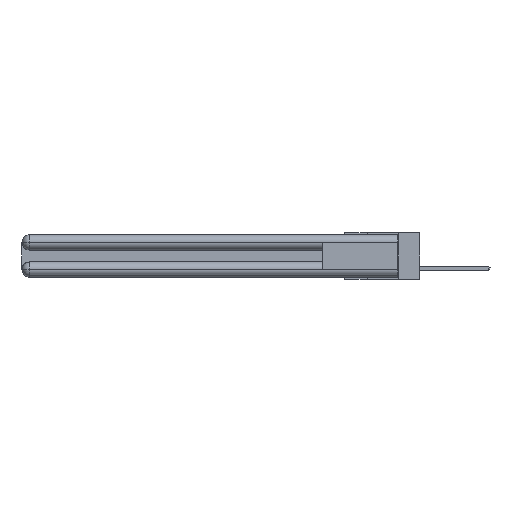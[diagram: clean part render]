
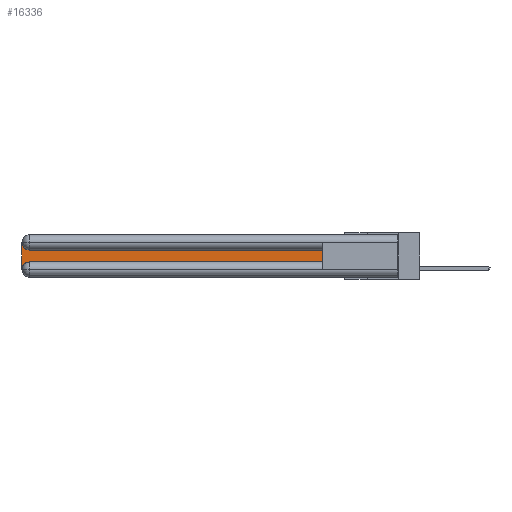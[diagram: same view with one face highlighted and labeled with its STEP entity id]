
A CAD part, left-side view. The second image highlights one B-rep face of the part: STEP entity #16336.
In plain terms, the highlighted planar face has unit normal (-1, 0, 0).
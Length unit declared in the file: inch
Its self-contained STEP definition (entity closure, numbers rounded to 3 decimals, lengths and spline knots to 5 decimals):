
#939 = VERTEX_POINT ( 'NONE', #7410 ) ;
#1721 = EDGE_CURVE ( 'NONE', #10157, #14634, #21906, .T. ) ;
#2072 = AXIS2_PLACEMENT_3D ( 'NONE', #21760, #19560, #8118 ) ;
#2104 = VERTEX_POINT ( 'NONE', #8947 ) ;
#2457 = VECTOR ( 'NONE', #24616, 39.37008 ) ;
#3689 = EDGE_LOOP ( 'NONE', ( #20193, #21967, #5775, #28191, #15033, #26736 ) ) ;
#3956 = EDGE_CURVE ( 'NONE', #939, #10157, #23600, .T. ) ;
#5775 = ORIENTED_EDGE ( 'NONE', *, *, #11467, .T. ) ;
#7410 = CARTESIAN_POINT ( 'NONE',  ( 0.075, 2.94, -0.2175 ) ) ;
#8118 = DIRECTION ( 'NONE',  ( 0., 0., -1. ) ) ;
#8134 = CARTESIAN_POINT ( 'NONE',  ( 0.075, 0.6, -0.1225 ) ) ;
#8425 = VERTEX_POINT ( 'NONE', #16467 ) ;
#8947 = CARTESIAN_POINT ( 'NONE',  ( 0.075, 3., -0.0625 ) ) ;
#10157 = VERTEX_POINT ( 'NONE', #27084 ) ;
#11119 = VECTOR ( 'NONE', #19125, 39.37008 ) ;
#11467 = EDGE_CURVE ( 'NONE', #2104, #8425, #17128, .T. ) ;
#12476 = AXIS2_PLACEMENT_3D ( 'NONE', #21191, #23612, #19287 ) ;
#13942 = VERTEX_POINT ( 'NONE', #28462 ) ;
#14634 = VERTEX_POINT ( 'NONE', #8134 ) ;
#15033 = ORIENTED_EDGE ( 'NONE', *, *, #3956, .T. ) ;
#15113 = CARTESIAN_POINT ( 'NONE',  ( 0.075, 3., -0.1225 ) ) ;
#15342 = EDGE_CURVE ( 'NONE', #8425, #939, #21113, .T. ) ;
#15667 = VECTOR ( 'NONE', #25379, 39.37008 ) ;
#16336 = ADVANCED_FACE ( 'NONE', ( #28320 ), #28887, .F. ) ;
#16467 = CARTESIAN_POINT ( 'NONE',  ( 0.075, 3., -0.2775 ) ) ;
#17128 = LINE ( 'NONE', #23083, #15667 ) ;
#17591 = CARTESIAN_POINT ( 'NONE',  ( 0.075, 0.6, -0.2175 ) ) ;
#19125 = DIRECTION ( 'NONE',  ( 0., 0., 1. ) ) ;
#19287 = DIRECTION ( 'NONE',  ( 0., 0., -1. ) ) ;
#19548 = VECTOR ( 'NONE', #29586, 39.37008 ) ;
#19560 = DIRECTION ( 'NONE',  ( 1., 0., 0. ) ) ;
#20193 = ORIENTED_EDGE ( 'NONE', *, *, #24172, .T. ) ;
#20629 = EDGE_CURVE ( 'NONE', #13942, #2104, #27631, .T. ) ;
#20967 = LINE ( 'NONE', #25072, #19548 ) ;
#21113 = CIRCLE ( 'NONE', #2072, 0.06 ) ;
#21191 = CARTESIAN_POINT ( 'NONE',  ( 0.075, 2.94, -0.0625 ) ) ;
#21760 = CARTESIAN_POINT ( 'NONE',  ( 0.075, 2.94, -0.2775 ) ) ;
#21906 = LINE ( 'NONE', #27532, #11119 ) ;
#21967 = ORIENTED_EDGE ( 'NONE', *, *, #20629, .T. ) ;
#22059 = DIRECTION ( 'NONE',  ( 1., 0., 0. ) ) ;
#23083 = CARTESIAN_POINT ( 'NONE',  ( 0.075, 3., -0.2175 ) ) ;
#23600 = LINE ( 'NONE', #17591, #2457 ) ;
#23612 = DIRECTION ( 'NONE',  ( 1., 0., 0. ) ) ;
#24172 = EDGE_CURVE ( 'NONE', #14634, #13942, #20967, .T. ) ;
#24381 = DIRECTION ( 'NONE',  ( 0., 0., -1. ) ) ;
#24616 = DIRECTION ( 'NONE',  ( 0., -1., 0. ) ) ;
#25072 = CARTESIAN_POINT ( 'NONE',  ( 0.075, 0.6, -0.1225 ) ) ;
#25379 = DIRECTION ( 'NONE',  ( 0., 0., -1. ) ) ;
#26736 = ORIENTED_EDGE ( 'NONE', *, *, #1721, .T. ) ;
#27084 = CARTESIAN_POINT ( 'NONE',  ( 0.075, 0.6, -0.2175 ) ) ;
#27532 = CARTESIAN_POINT ( 'NONE',  ( 0.075, 0.6, -0.2175 ) ) ;
#27631 = CIRCLE ( 'NONE', #12476, 0.06 ) ;
#28191 = ORIENTED_EDGE ( 'NONE', *, *, #15342, .T. ) ;
#28320 = FACE_OUTER_BOUND ( 'NONE', #3689, .T. ) ;
#28462 = CARTESIAN_POINT ( 'NONE',  ( 0.075, 2.94, -0.1225 ) ) ;
#28887 = PLANE ( 'NONE',  #29173 ) ;
#29173 = AXIS2_PLACEMENT_3D ( 'NONE', #15113, #22059, #24381 ) ;
#29586 = DIRECTION ( 'NONE',  ( 0., 1., 0. ) ) ;
